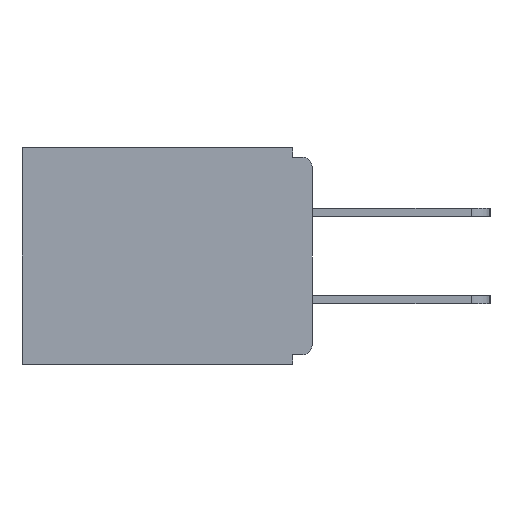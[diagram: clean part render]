
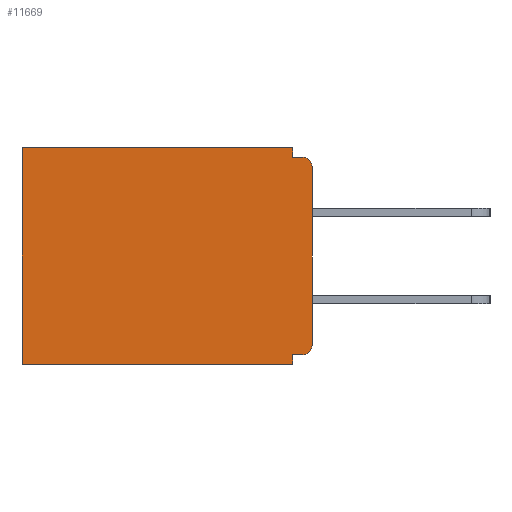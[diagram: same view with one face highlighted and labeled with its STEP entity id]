
A CAD part, left-side view. The second image highlights one B-rep face of the part: STEP entity #11669.
In plain terms, the highlighted planar face has unit normal (-1, 0, 0).
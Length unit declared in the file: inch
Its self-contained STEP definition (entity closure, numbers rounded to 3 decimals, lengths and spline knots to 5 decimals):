
#305 = ORIENTED_EDGE ( 'NONE', *, *, #16347, .T. ) ;
#605 = CARTESIAN_POINT ( 'NONE',  ( 0.298, 0., 0. ) ) ;
#637 = LINE ( 'NONE', #4192, #16554 ) ;
#646 = VECTOR ( 'NONE', #15529, 39.37008 ) ;
#677 = CARTESIAN_POINT ( 'NONE',  ( 0.298, 0.015, -0.015 ) ) ;
#776 = EDGE_LOOP ( 'NONE', ( #305, #5850, #3367, #15622, #3344, #14566, #3240, #19664, #9106, #14922 ) ) ;
#985 = EDGE_CURVE ( 'NONE', #19965, #11774, #21704, .T. ) ;
#1611 = VERTEX_POINT ( 'NONE', #677 ) ;
#1818 = CARTESIAN_POINT ( 'NONE',  ( 0.298, 0., -0.328 ) ) ;
#2141 = VECTOR ( 'NONE', #8602, 39.37008 ) ;
#2549 = DIRECTION ( 'NONE',  ( 0., 0., -1. ) ) ;
#2839 = CARTESIAN_POINT ( 'NONE',  ( 0.298, 0., -0.343 ) ) ;
#2923 = CARTESIAN_POINT ( 'NONE',  ( 0.298, 0.031, -0.343 ) ) ;
#3069 = EDGE_CURVE ( 'NONE', #8638, #21600, #637, .T. ) ;
#3240 = ORIENTED_EDGE ( 'NONE', *, *, #6313, .F. ) ;
#3344 = ORIENTED_EDGE ( 'NONE', *, *, #3069, .T. ) ;
#3367 = ORIENTED_EDGE ( 'NONE', *, *, #20971, .F. ) ;
#3387 = DIRECTION ( 'NONE',  ( -1., 0., 0. ) ) ;
#3469 = CARTESIAN_POINT ( 'NONE',  ( 0.298, 0.015, -0.313 ) ) ;
#4020 = LINE ( 'NONE', #2839, #4314 ) ;
#4060 = CARTESIAN_POINT ( 'NONE',  ( 0.298, 0., -0.313 ) ) ;
#4192 = CARTESIAN_POINT ( 'NONE',  ( 0.298, 0.46, 0. ) ) ;
#4251 = AXIS2_PLACEMENT_3D ( 'NONE', #5595, #7410, #12940 ) ;
#4314 = VECTOR ( 'NONE', #4627, 39.37008 ) ;
#4327 = LINE ( 'NONE', #6023, #12138 ) ;
#4571 = LINE ( 'NONE', #605, #20203 ) ;
#4627 = DIRECTION ( 'NONE',  ( 0., 1., 0. ) ) ;
#4803 = CARTESIAN_POINT ( 'NONE',  ( 0.298, 0.015, -0.328 ) ) ;
#4980 = CARTESIAN_POINT ( 'NONE',  ( 0.298, 0., -0.03 ) ) ;
#5595 = CARTESIAN_POINT ( 'NONE',  ( 0.298, 0.015, -0.03 ) ) ;
#5645 = EDGE_CURVE ( 'NONE', #22908, #1611, #4327, .T. ) ;
#5850 = ORIENTED_EDGE ( 'NONE', *, *, #5645, .F. ) ;
#6023 = CARTESIAN_POINT ( 'NONE',  ( 0.298, 0., -0.015 ) ) ;
#6211 = EDGE_CURVE ( 'NONE', #19247, #8638, #4571, .T. ) ;
#6276 = DIRECTION ( 'NONE',  ( 1., 0., 0. ) ) ;
#6313 = EDGE_CURVE ( 'NONE', #7543, #10352, #12671, .T. ) ;
#6527 = VECTOR ( 'NONE', #8283, 39.37008 ) ;
#7410 = DIRECTION ( 'NONE',  ( -1., 0., 0. ) ) ;
#7516 = CARTESIAN_POINT ( 'NONE',  ( 0.298, 0.031, -0.343 ) ) ;
#7543 = VERTEX_POINT ( 'NONE', #11896 ) ;
#7949 = PLANE ( 'NONE',  #9399 ) ;
#7971 = LINE ( 'NONE', #1818, #6527 ) ;
#8283 = DIRECTION ( 'NONE',  ( 0., 1., 0. ) ) ;
#8475 = CARTESIAN_POINT ( 'NONE',  ( 0.298, 0.031, -0.015 ) ) ;
#8602 = DIRECTION ( 'NONE',  ( 0., 0., -1. ) ) ;
#8638 = VERTEX_POINT ( 'NONE', #18408 ) ;
#8984 = DIRECTION ( 'NONE',  ( 0., 0., -1. ) ) ;
#9106 = ORIENTED_EDGE ( 'NONE', *, *, #21745, .T. ) ;
#9399 = AXIS2_PLACEMENT_3D ( 'NONE', #20422, #6276, #20493 ) ;
#9453 = VERTEX_POINT ( 'NONE', #4803 ) ;
#10352 = VERTEX_POINT ( 'NONE', #20184 ) ;
#11669 = ADVANCED_FACE ( 'NONE', ( #19720 ), #7949, .F. ) ;
#11774 = VERTEX_POINT ( 'NONE', #4060 ) ;
#11896 = CARTESIAN_POINT ( 'NONE',  ( 0.298, 0.031, -0.328 ) ) ;
#12138 = VECTOR ( 'NONE', #16794, 39.37008 ) ;
#12307 = EDGE_CURVE ( 'NONE', #9453, #7543, #7971, .T. ) ;
#12508 = EDGE_CURVE ( 'NONE', #10352, #21600, #4020, .T. ) ;
#12671 = LINE ( 'NONE', #2923, #646 ) ;
#12940 = DIRECTION ( 'NONE',  ( 0., 0., -1. ) ) ;
#13106 = DIRECTION ( 'NONE',  ( 0., 0., -1. ) ) ;
#13561 = CIRCLE ( 'NONE', #4251, 0.015 ) ;
#13646 = CARTESIAN_POINT ( 'NONE',  ( 0.298, 0.031, 0. ) ) ;
#14566 = ORIENTED_EDGE ( 'NONE', *, *, #12508, .F. ) ;
#14883 = AXIS2_PLACEMENT_3D ( 'NONE', #3469, #3387, #8984 ) ;
#14922 = ORIENTED_EDGE ( 'NONE', *, *, #985, .F. ) ;
#15311 = VECTOR ( 'NONE', #13106, 39.37008 ) ;
#15529 = DIRECTION ( 'NONE',  ( 0., 0., -1. ) ) ;
#15622 = ORIENTED_EDGE ( 'NONE', *, *, #6211, .T. ) ;
#16347 = EDGE_CURVE ( 'NONE', #19965, #1611, #13561, .T. ) ;
#16554 = VECTOR ( 'NONE', #2549, 39.37008 ) ;
#16697 = CIRCLE ( 'NONE', #14883, 0.015 ) ;
#16794 = DIRECTION ( 'NONE',  ( 0., -1., 0. ) ) ;
#17410 = CARTESIAN_POINT ( 'NONE',  ( 0.298, 0., 0. ) ) ;
#18408 = CARTESIAN_POINT ( 'NONE',  ( 0.298, 0.46, 0. ) ) ;
#19247 = VERTEX_POINT ( 'NONE', #13646 ) ;
#19664 = ORIENTED_EDGE ( 'NONE', *, *, #12307, .F. ) ;
#19720 = FACE_OUTER_BOUND ( 'NONE', #776, .T. ) ;
#19965 = VERTEX_POINT ( 'NONE', #4980 ) ;
#20049 = DIRECTION ( 'NONE',  ( 0., 1., 0. ) ) ;
#20097 = LINE ( 'NONE', #7516, #15311 ) ;
#20184 = CARTESIAN_POINT ( 'NONE',  ( 0.298, 0.031, -0.343 ) ) ;
#20203 = VECTOR ( 'NONE', #20049, 39.37008 ) ;
#20339 = CARTESIAN_POINT ( 'NONE',  ( 0.298, 0.46, -0.343 ) ) ;
#20422 = CARTESIAN_POINT ( 'NONE',  ( 0.298, 0., 0. ) ) ;
#20493 = DIRECTION ( 'NONE',  ( 0., 0., -1. ) ) ;
#20971 = EDGE_CURVE ( 'NONE', #19247, #22908, #20097, .T. ) ;
#21600 = VERTEX_POINT ( 'NONE', #20339 ) ;
#21704 = LINE ( 'NONE', #17410, #2141 ) ;
#21745 = EDGE_CURVE ( 'NONE', #9453, #11774, #16697, .T. ) ;
#22908 = VERTEX_POINT ( 'NONE', #8475 ) ;
